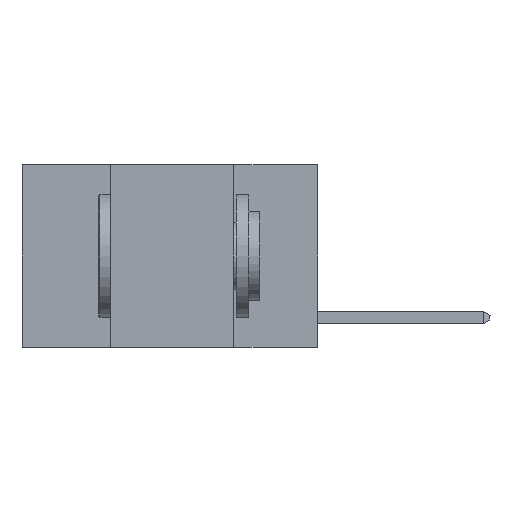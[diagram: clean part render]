
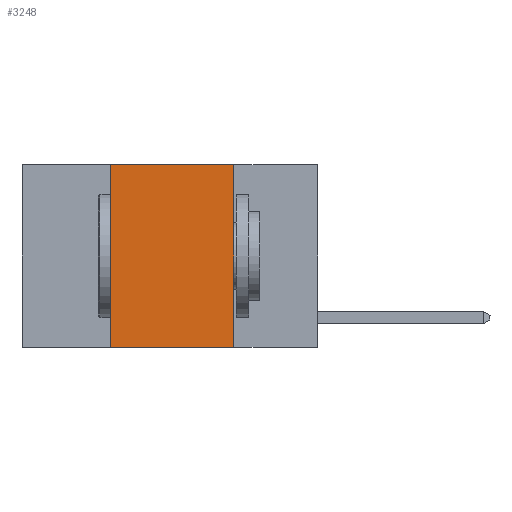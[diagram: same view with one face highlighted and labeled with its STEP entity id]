
A CAD part, left-side view. The second image highlights one B-rep face of the part: STEP entity #3248.
In plain terms, the highlighted planar face has unit normal (-1, 0, 0).
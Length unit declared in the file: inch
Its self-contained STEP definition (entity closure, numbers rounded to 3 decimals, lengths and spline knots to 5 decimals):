
#906 = VERTEX_POINT ( 'NONE', #3177 ) ;
#1133 = VERTEX_POINT ( 'NONE', #5786 ) ;
#1474 = VERTEX_POINT ( 'NONE', #7711 ) ;
#1508 = VECTOR ( 'NONE', #2361, 39.37008 ) ;
#2348 = EDGE_CURVE ( 'NONE', #1133, #5907, #4902, .T. ) ;
#2361 = DIRECTION ( 'NONE',  ( 0., -1., 0. ) ) ;
#2735 = CARTESIAN_POINT ( 'NONE',  ( 0., 0.6, -0.37 ) ) ;
#2930 = VECTOR ( 'NONE', #8070, 39.37008 ) ;
#3048 = LINE ( 'NONE', #10896, #9672 ) ;
#3177 = CARTESIAN_POINT ( 'NONE',  ( 0., 0.42, 0. ) ) ;
#3190 = EDGE_CURVE ( 'NONE', #1133, #906, #3048, .T. ) ;
#3248 = ADVANCED_FACE ( 'NONE', ( #14665 ), #9852, .F. ) ;
#3352 = LINE ( 'NONE', #6857, #2930 ) ;
#3588 = DIRECTION ( 'NONE',  ( 0., 0., 1. ) ) ;
#3706 = DIRECTION ( 'NONE',  ( 1., 0., 0. ) ) ;
#4415 = ORIENTED_EDGE ( 'NONE', *, *, #12560, .F. ) ;
#4902 = LINE ( 'NONE', #2735, #1508 ) ;
#5786 = CARTESIAN_POINT ( 'NONE',  ( 0., 0.42, -0.37 ) ) ;
#5792 = EDGE_CURVE ( 'NONE', #1474, #5907, #3352, .T. ) ;
#5907 = VERTEX_POINT ( 'NONE', #7075 ) ;
#6857 = CARTESIAN_POINT ( 'NONE',  ( 0., 0.17, 0. ) ) ;
#7075 = CARTESIAN_POINT ( 'NONE',  ( 0., 0.17, -0.37 ) ) ;
#7351 = VECTOR ( 'NONE', #12526, 39.37008 ) ;
#7369 = ORIENTED_EDGE ( 'NONE', *, *, #5792, .F. ) ;
#7711 = CARTESIAN_POINT ( 'NONE',  ( 0., 0.17, 0. ) ) ;
#7743 = ORIENTED_EDGE ( 'NONE', *, *, #3190, .F. ) ;
#8070 = DIRECTION ( 'NONE',  ( 0., 0., -1. ) ) ;
#8982 = EDGE_LOOP ( 'NONE', ( #7369, #4415, #7743, #13893 ) ) ;
#9047 = CARTESIAN_POINT ( 'NONE',  ( 0., 0.6, 0. ) ) ;
#9672 = VECTOR ( 'NONE', #3588, 39.37008 ) ;
#9852 = PLANE ( 'NONE',  #9884 ) ;
#9884 = AXIS2_PLACEMENT_3D ( 'NONE', #10994, #3706, #12166 ) ;
#10846 = LINE ( 'NONE', #9047, #7351 ) ;
#10896 = CARTESIAN_POINT ( 'NONE',  ( 0., 0.42, 0. ) ) ;
#10994 = CARTESIAN_POINT ( 'NONE',  ( 0., 0.6, 0. ) ) ;
#12166 = DIRECTION ( 'NONE',  ( 0., 0., -1. ) ) ;
#12526 = DIRECTION ( 'NONE',  ( 0., -1., 0. ) ) ;
#12560 = EDGE_CURVE ( 'NONE', #906, #1474, #10846, .T. ) ;
#13893 = ORIENTED_EDGE ( 'NONE', *, *, #2348, .T. ) ;
#14665 = FACE_OUTER_BOUND ( 'NONE', #8982, .T. ) ;
